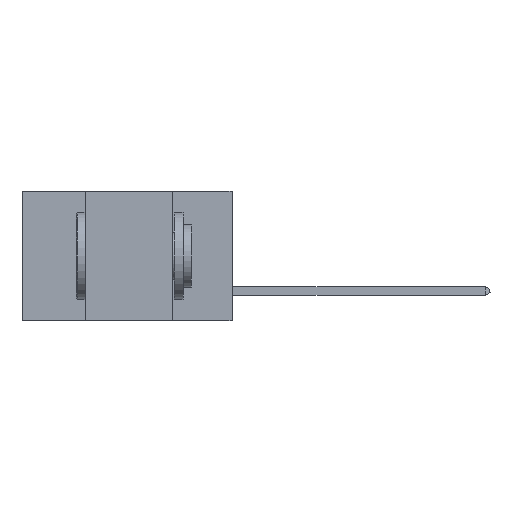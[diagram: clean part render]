
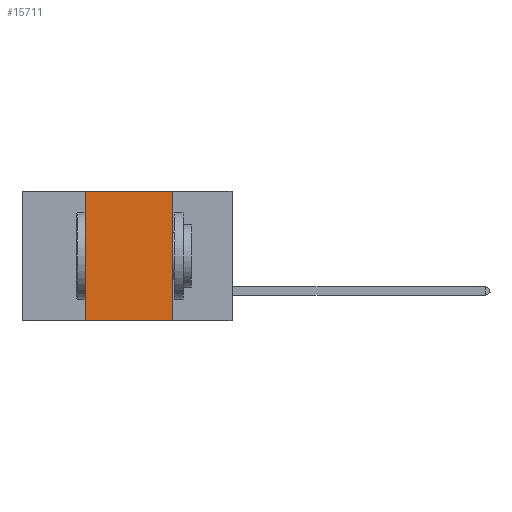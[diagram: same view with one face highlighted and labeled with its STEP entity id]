
A CAD part, left-side view. The second image highlights one B-rep face of the part: STEP entity #15711.
In plain terms, the highlighted planar face has unit normal (-1, 0, 0).
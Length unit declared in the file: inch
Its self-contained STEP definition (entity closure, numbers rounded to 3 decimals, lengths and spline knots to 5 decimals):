
#969 = EDGE_CURVE ( 'NONE', #21879, #28963, #22539, .T. ) ;
#1810 = CARTESIAN_POINT ( 'NONE',  ( 0., 0.42, 0. ) ) ;
#2137 = EDGE_CURVE ( 'NONE', #9320, #21879, #20687, .T. ) ;
#3301 = CARTESIAN_POINT ( 'NONE',  ( 0., 0.6, -0.37 ) ) ;
#4014 = VECTOR ( 'NONE', #16642, 39.37008 ) ;
#4411 = CARTESIAN_POINT ( 'NONE',  ( 0., 0.17, -0.37 ) ) ;
#5667 = DIRECTION ( 'NONE',  ( 0., 0., -1. ) ) ;
#6305 = AXIS2_PLACEMENT_3D ( 'NONE', #29116, #17429, #22249 ) ;
#6716 = CARTESIAN_POINT ( 'NONE',  ( 0., 0.42, -0.37 ) ) ;
#7578 = EDGE_CURVE ( 'NONE', #16821, #9320, #20656, .T. ) ;
#8035 = VECTOR ( 'NONE', #5667, 39.37008 ) ;
#9320 = VERTEX_POINT ( 'NONE', #24980 ) ;
#9522 = DIRECTION ( 'NONE',  ( 0., 0., 1. ) ) ;
#13146 = ORIENTED_EDGE ( 'NONE', *, *, #7578, .F. ) ;
#13180 = ORIENTED_EDGE ( 'NONE', *, *, #17131, .T. ) ;
#13988 = ORIENTED_EDGE ( 'NONE', *, *, #2137, .F. ) ;
#14785 = FACE_OUTER_BOUND ( 'NONE', #28598, .T. ) ;
#15711 = ADVANCED_FACE ( 'NONE', ( #14785 ), #21949, .F. ) ;
#16642 = DIRECTION ( 'NONE',  ( 0., -1., 0. ) ) ;
#16821 = VERTEX_POINT ( 'NONE', #6716 ) ;
#17131 = EDGE_CURVE ( 'NONE', #16821, #28963, #23525, .T. ) ;
#17429 = DIRECTION ( 'NONE',  ( 1., 0., 0. ) ) ;
#18243 = VECTOR ( 'NONE', #28370, 39.37008 ) ;
#19285 = CARTESIAN_POINT ( 'NONE',  ( 0., 0.17, 0. ) ) ;
#20317 = VECTOR ( 'NONE', #9522, 39.37008 ) ;
#20656 = LINE ( 'NONE', #1810, #20317 ) ;
#20687 = LINE ( 'NONE', #21171, #4014 ) ;
#21171 = CARTESIAN_POINT ( 'NONE',  ( 0., 0.6, 0. ) ) ;
#21879 = VERTEX_POINT ( 'NONE', #23745 ) ;
#21949 = PLANE ( 'NONE',  #6305 ) ;
#22249 = DIRECTION ( 'NONE',  ( 0., 0., -1. ) ) ;
#22539 = LINE ( 'NONE', #19285, #8035 ) ;
#23109 = ORIENTED_EDGE ( 'NONE', *, *, #969, .F. ) ;
#23525 = LINE ( 'NONE', #3301, #18243 ) ;
#23745 = CARTESIAN_POINT ( 'NONE',  ( 0., 0.17, 0. ) ) ;
#24980 = CARTESIAN_POINT ( 'NONE',  ( 0., 0.42, 0. ) ) ;
#28370 = DIRECTION ( 'NONE',  ( 0., -1., 0. ) ) ;
#28598 = EDGE_LOOP ( 'NONE', ( #23109, #13988, #13146, #13180 ) ) ;
#28963 = VERTEX_POINT ( 'NONE', #4411 ) ;
#29116 = CARTESIAN_POINT ( 'NONE',  ( 0., 0.6, 0. ) ) ;
